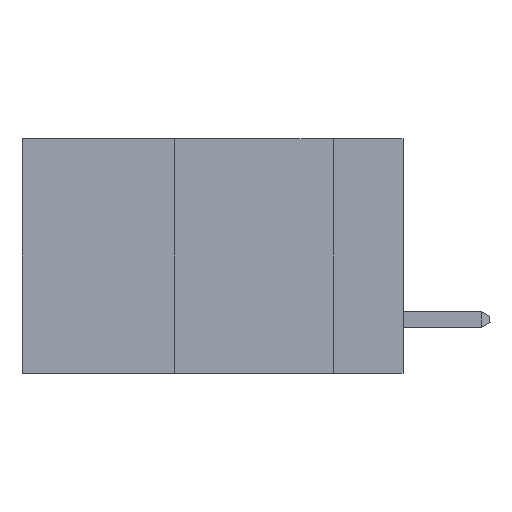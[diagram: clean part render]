
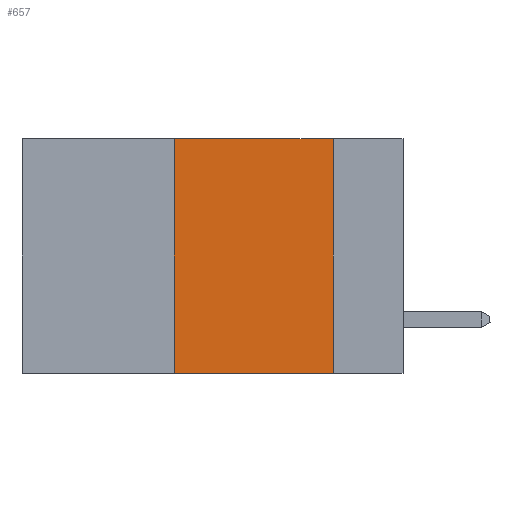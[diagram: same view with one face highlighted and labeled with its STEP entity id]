
A CAD part, left-side view. The second image highlights one B-rep face of the part: STEP entity #657.
In plain terms, the highlighted planar face has unit normal (-1, 0, 0).
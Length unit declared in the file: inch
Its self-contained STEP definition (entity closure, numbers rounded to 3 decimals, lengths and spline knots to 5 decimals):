
#657 = ADVANCED_FACE ( 'NONE', ( #29330 ), #17921, .F. ) ;
#2669 = EDGE_LOOP ( 'NONE', ( #26748, #19986, #28557, #15345 ) ) ;
#3536 = DIRECTION ( 'NONE',  ( 0., -1., 0. ) ) ;
#3985 = LINE ( 'NONE', #20857, #31318 ) ;
#4747 = CARTESIAN_POINT ( 'NONE',  ( 0., 0.36, 0. ) ) ;
#6235 = AXIS2_PLACEMENT_3D ( 'NONE', #31563, #34246, #18045 ) ;
#7243 = DIRECTION ( 'NONE',  ( 0., 0., -1. ) ) ;
#8019 = EDGE_CURVE ( 'NONE', #32157, #25669, #32315, .T. ) ;
#11651 = CARTESIAN_POINT ( 'NONE',  ( 0., 0.6, -0.37 ) ) ;
#11714 = EDGE_CURVE ( 'NONE', #34799, #25669, #3985, .T. ) ;
#12929 = VECTOR ( 'NONE', #34822, 39.37008 ) ;
#13826 = EDGE_CURVE ( 'NONE', #32157, #32661, #32841, .T. ) ;
#14394 = DIRECTION ( 'NONE',  ( 0., -1., 0. ) ) ;
#14708 = VECTOR ( 'NONE', #3536, 39.37008 ) ;
#15345 = ORIENTED_EDGE ( 'NONE', *, *, #8019, .T. ) ;
#17921 = PLANE ( 'NONE',  #6235 ) ;
#18045 = DIRECTION ( 'NONE',  ( 0., 0., -1. ) ) ;
#19986 = ORIENTED_EDGE ( 'NONE', *, *, #29002, .F. ) ;
#20857 = CARTESIAN_POINT ( 'NONE',  ( 0., 0.11, 0. ) ) ;
#23600 = LINE ( 'NONE', #33597, #14708 ) ;
#25669 = VERTEX_POINT ( 'NONE', #34079 ) ;
#26748 = ORIENTED_EDGE ( 'NONE', *, *, #11714, .F. ) ;
#28557 = ORIENTED_EDGE ( 'NONE', *, *, #13826, .F. ) ;
#29002 = EDGE_CURVE ( 'NONE', #32661, #34799, #23600, .T. ) ;
#29330 = FACE_OUTER_BOUND ( 'NONE', #2669, .T. ) ;
#30975 = CARTESIAN_POINT ( 'NONE',  ( 0., 0.11, 0. ) ) ;
#31318 = VECTOR ( 'NONE', #7243, 39.37008 ) ;
#31563 = CARTESIAN_POINT ( 'NONE',  ( 0., 0.6, 0. ) ) ;
#32157 = VERTEX_POINT ( 'NONE', #32695 ) ;
#32315 = LINE ( 'NONE', #11651, #33152 ) ;
#32661 = VERTEX_POINT ( 'NONE', #4747 ) ;
#32695 = CARTESIAN_POINT ( 'NONE',  ( 0., 0.36, -0.37 ) ) ;
#32841 = LINE ( 'NONE', #34942, #12929 ) ;
#33152 = VECTOR ( 'NONE', #14394, 39.37008 ) ;
#33597 = CARTESIAN_POINT ( 'NONE',  ( 0., 0.6, 0. ) ) ;
#34079 = CARTESIAN_POINT ( 'NONE',  ( 0., 0.11, -0.37 ) ) ;
#34246 = DIRECTION ( 'NONE',  ( 1., 0., 0. ) ) ;
#34799 = VERTEX_POINT ( 'NONE', #30975 ) ;
#34822 = DIRECTION ( 'NONE',  ( 0., 0., 1. ) ) ;
#34942 = CARTESIAN_POINT ( 'NONE',  ( 0., 0.36, 0. ) ) ;
